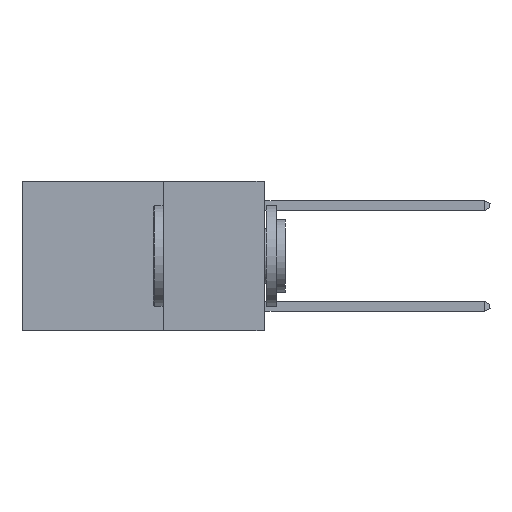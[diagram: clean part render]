
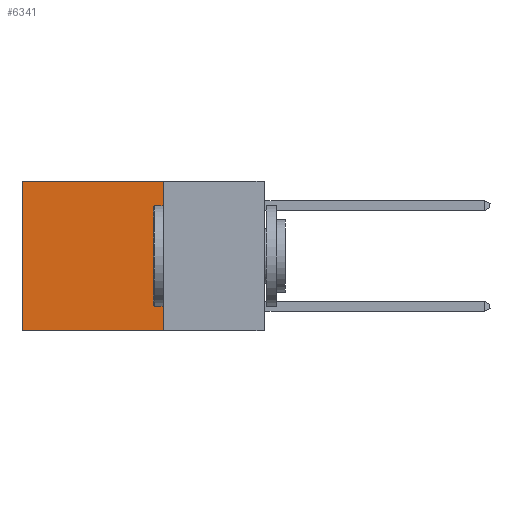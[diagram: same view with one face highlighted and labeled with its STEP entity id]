
A CAD part, left-side view. The second image highlights one B-rep face of the part: STEP entity #6341.
In plain terms, the highlighted planar face has unit normal (-1, 0, 0).
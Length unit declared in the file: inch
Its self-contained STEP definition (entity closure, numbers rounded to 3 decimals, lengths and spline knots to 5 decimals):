
#799 = ORIENTED_EDGE ( 'NONE', *, *, #9022, .F. ) ;
#997 = ORIENTED_EDGE ( 'NONE', *, *, #10313, .T. ) ;
#1597 = DIRECTION ( 'NONE',  ( 0., 0., -1. ) ) ;
#2908 = CARTESIAN_POINT ( 'NONE',  ( 0.2625, 0.25, 0. ) ) ;
#2970 = VERTEX_POINT ( 'NONE', #23803 ) ;
#3633 = ORIENTED_EDGE ( 'NONE', *, *, #15921, .T. ) ;
#3824 = EDGE_LOOP ( 'NONE', ( #997, #799, #21860, #3633 ) ) ;
#3971 = VECTOR ( 'NONE', #4545, 39.37008 ) ;
#4539 = VECTOR ( 'NONE', #8878, 39.37008 ) ;
#4545 = DIRECTION ( 'NONE',  ( 0., 0., -1. ) ) ;
#5298 = CARTESIAN_POINT ( 'NONE',  ( 0.2625, 0.25, -0.37 ) ) ;
#5554 = DIRECTION ( 'NONE',  ( 0., 1., 0. ) ) ;
#6341 = ADVANCED_FACE ( 'NONE', ( #23407 ), #13540, .F. ) ;
#6347 = CARTESIAN_POINT ( 'NONE',  ( 0.2625, 0.6, -0.37 ) ) ;
#6603 = VECTOR ( 'NONE', #5554, 39.37008 ) ;
#7662 = LINE ( 'NONE', #5298, #6603 ) ;
#8878 = DIRECTION ( 'NONE',  ( 0., 0., -1. ) ) ;
#9022 = EDGE_CURVE ( 'NONE', #12757, #24465, #7662, .T. ) ;
#10128 = VECTOR ( 'NONE', #10896, 39.37008 ) ;
#10313 = EDGE_CURVE ( 'NONE', #24383, #24465, #14509, .T. ) ;
#10896 = DIRECTION ( 'NONE',  ( 0., 1., 0. ) ) ;
#11156 = LINE ( 'NONE', #2908, #10128 ) ;
#11432 = CARTESIAN_POINT ( 'NONE',  ( 0.2625, 0.25, 0. ) ) ;
#12757 = VERTEX_POINT ( 'NONE', #21790 ) ;
#13004 = CARTESIAN_POINT ( 'NONE',  ( 0.2625, 0.6, 0. ) ) ;
#13540 = PLANE ( 'NONE',  #18596 ) ;
#14509 = LINE ( 'NONE', #16216, #3971 ) ;
#14897 = CARTESIAN_POINT ( 'NONE',  ( 0.2625, 0.25, 0. ) ) ;
#15921 = EDGE_CURVE ( 'NONE', #2970, #24383, #11156, .T. ) ;
#16216 = CARTESIAN_POINT ( 'NONE',  ( 0.2625, 0.6, 0. ) ) ;
#17098 = DIRECTION ( 'NONE',  ( 1., 0., 0. ) ) ;
#18596 = AXIS2_PLACEMENT_3D ( 'NONE', #11432, #17098, #1597 ) ;
#20940 = LINE ( 'NONE', #14897, #4539 ) ;
#21790 = CARTESIAN_POINT ( 'NONE',  ( 0.2625, 0.25, -0.37 ) ) ;
#21860 = ORIENTED_EDGE ( 'NONE', *, *, #25154, .F. ) ;
#23407 = FACE_OUTER_BOUND ( 'NONE', #3824, .T. ) ;
#23803 = CARTESIAN_POINT ( 'NONE',  ( 0.2625, 0.25, 0. ) ) ;
#24383 = VERTEX_POINT ( 'NONE', #13004 ) ;
#24465 = VERTEX_POINT ( 'NONE', #6347 ) ;
#25154 = EDGE_CURVE ( 'NONE', #2970, #12757, #20940, .T. ) ;
